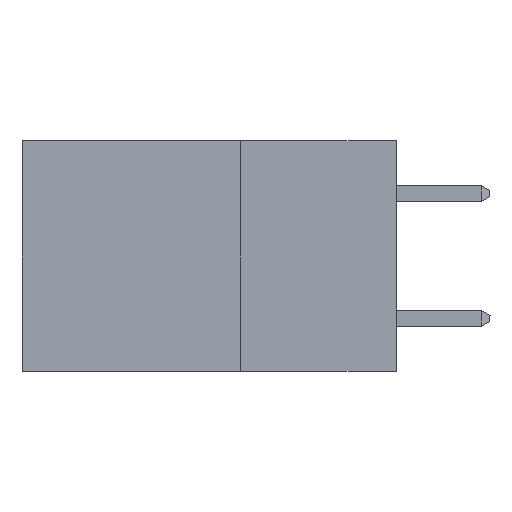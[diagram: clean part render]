
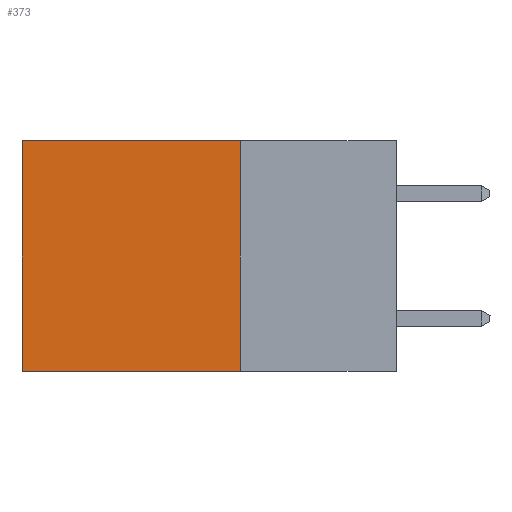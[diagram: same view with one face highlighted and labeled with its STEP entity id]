
A CAD part, left-side view. The second image highlights one B-rep face of the part: STEP entity #373.
In plain terms, the highlighted planar face has unit normal (-1, 0, 0).
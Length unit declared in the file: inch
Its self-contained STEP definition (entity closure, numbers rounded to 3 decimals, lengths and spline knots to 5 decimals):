
#8 = LINE ( 'NONE', #3864, #12969 ) ;
#373 = ADVANCED_FACE ( 'NONE', ( #5350 ), #4118, .F. ) ;
#615 = EDGE_CURVE ( 'NONE', #10829, #12885, #11006, .T. ) ;
#646 = VERTEX_POINT ( 'NONE', #9103 ) ;
#1830 = VECTOR ( 'NONE', #11793, 39.37008 ) ;
#1949 = CARTESIAN_POINT ( 'NONE',  ( 0.2615, 0.25, -0.37 ) ) ;
#2330 = ORIENTED_EDGE ( 'NONE', *, *, #2467, .F. ) ;
#2467 = EDGE_CURVE ( 'NONE', #12885, #646, #5082, .T. ) ;
#2929 = DIRECTION ( 'NONE',  ( 0., 1., 0. ) ) ;
#3024 = EDGE_CURVE ( 'NONE', #10829, #8267, #9660, .T. ) ;
#3864 = CARTESIAN_POINT ( 'NONE',  ( 0.2615, 0.6, -0.37 ) ) ;
#4021 = DIRECTION ( 'NONE',  ( 0., 0., -1. ) ) ;
#4077 = DIRECTION ( 'NONE',  ( 1., 0., 0. ) ) ;
#4118 = PLANE ( 'NONE',  #10273 ) ;
#4736 = VECTOR ( 'NONE', #2929, 39.37008 ) ;
#5082 = LINE ( 'NONE', #11398, #4736 ) ;
#5332 = VECTOR ( 'NONE', #12838, 39.37008 ) ;
#5350 = FACE_OUTER_BOUND ( 'NONE', #7080, .T. ) ;
#5413 = CARTESIAN_POINT ( 'NONE',  ( 0.2615, 0.25, 0. ) ) ;
#6515 = ORIENTED_EDGE ( 'NONE', *, *, #10999, .T. ) ;
#7080 = EDGE_LOOP ( 'NONE', ( #6515, #2330, #11938, #11913 ) ) ;
#7161 = CARTESIAN_POINT ( 'NONE',  ( 0.2615, 0.25, -0.37 ) ) ;
#8267 = VERTEX_POINT ( 'NONE', #8696 ) ;
#8289 = DIRECTION ( 'NONE',  ( 0., 0., -1. ) ) ;
#8696 = CARTESIAN_POINT ( 'NONE',  ( 0.2615, 0.6, 0. ) ) ;
#9103 = CARTESIAN_POINT ( 'NONE',  ( 0.2615, 0.6, -0.37 ) ) ;
#9333 = CARTESIAN_POINT ( 'NONE',  ( 0.2615, 0.25, -0.37 ) ) ;
#9660 = LINE ( 'NONE', #12436, #1830 ) ;
#10273 = AXIS2_PLACEMENT_3D ( 'NONE', #7161, #4077, #8289 ) ;
#10829 = VERTEX_POINT ( 'NONE', #5413 ) ;
#10999 = EDGE_CURVE ( 'NONE', #8267, #646, #8, .T. ) ;
#11006 = LINE ( 'NONE', #1949, #5332 ) ;
#11398 = CARTESIAN_POINT ( 'NONE',  ( 0.2615, 0.25, -0.37 ) ) ;
#11793 = DIRECTION ( 'NONE',  ( 0., 1., 0. ) ) ;
#11913 = ORIENTED_EDGE ( 'NONE', *, *, #3024, .T. ) ;
#11938 = ORIENTED_EDGE ( 'NONE', *, *, #615, .F. ) ;
#12436 = CARTESIAN_POINT ( 'NONE',  ( 0.2615, 0.25, 0. ) ) ;
#12838 = DIRECTION ( 'NONE',  ( 0., 0., -1. ) ) ;
#12885 = VERTEX_POINT ( 'NONE', #9333 ) ;
#12969 = VECTOR ( 'NONE', #4021, 39.37008 ) ;
